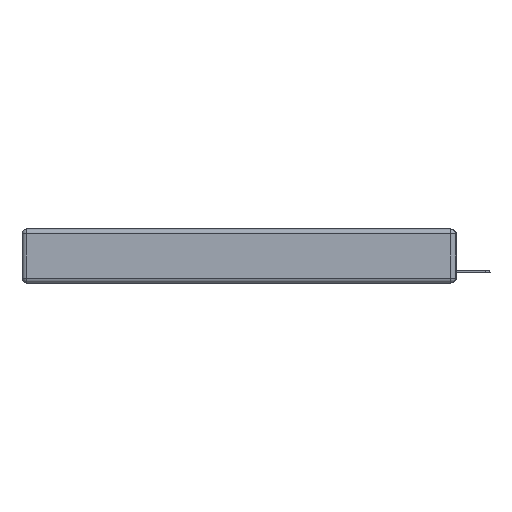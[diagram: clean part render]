
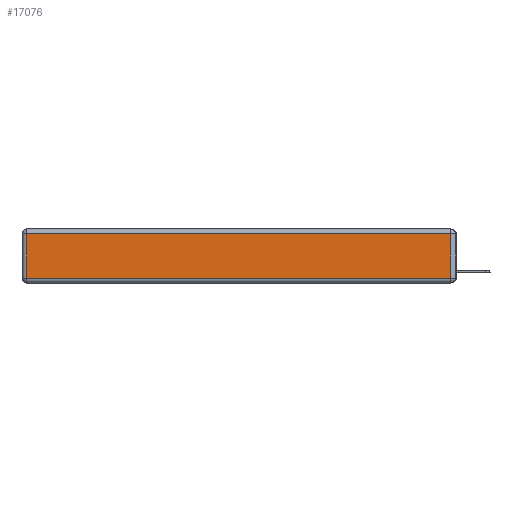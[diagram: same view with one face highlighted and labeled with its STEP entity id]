
A CAD part, left-side view. The second image highlights one B-rep face of the part: STEP entity #17076.
In plain terms, the highlighted planar face has unit normal (-1, 0, 0).
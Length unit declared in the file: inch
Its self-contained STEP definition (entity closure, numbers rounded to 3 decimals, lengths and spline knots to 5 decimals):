
#605 = CARTESIAN_POINT ( 'NONE',  ( 0., 2.72, -0.03 ) ) ;
#669 = EDGE_CURVE ( 'NONE', #10921, #11636, #18666, .T. ) ;
#800 = LINE ( 'NONE', #21331, #5895 ) ;
#1928 = LINE ( 'NONE', #9284, #22316 ) ;
#3323 = VECTOR ( 'NONE', #9651, 39.37008 ) ;
#4001 = DIRECTION ( 'NONE',  ( -1., 0., 0. ) ) ;
#5895 = VECTOR ( 'NONE', #8503, 39.37008 ) ;
#6489 = CARTESIAN_POINT ( 'NONE',  ( 0., 0.03, -0.313 ) ) ;
#7535 = EDGE_CURVE ( 'NONE', #11636, #9770, #1928, .T. ) ;
#7806 = LINE ( 'NONE', #19292, #3323 ) ;
#8338 = ORIENTED_EDGE ( 'NONE', *, *, #669, .T. ) ;
#8503 = DIRECTION ( 'NONE',  ( 0., 1., 0. ) ) ;
#9272 = CARTESIAN_POINT ( 'NONE',  ( 0., 0., -0.343 ) ) ;
#9284 = CARTESIAN_POINT ( 'NONE',  ( 0., 0.03, -0.343 ) ) ;
#9405 = DIRECTION ( 'NONE',  ( 0., 0., 1. ) ) ;
#9651 = DIRECTION ( 'NONE',  ( 0., 0., -1. ) ) ;
#9770 = VERTEX_POINT ( 'NONE', #18878 ) ;
#10065 = ORIENTED_EDGE ( 'NONE', *, *, #11985, .T. ) ;
#10921 = VERTEX_POINT ( 'NONE', #13803 ) ;
#11482 = DIRECTION ( 'NONE',  ( 0., 0., 1. ) ) ;
#11636 = VERTEX_POINT ( 'NONE', #6489 ) ;
#11985 = EDGE_CURVE ( 'NONE', #18352, #10921, #7806, .T. ) ;
#13312 = PLANE ( 'NONE',  #23325 ) ;
#13803 = CARTESIAN_POINT ( 'NONE',  ( 0., 2.72, -0.313 ) ) ;
#13859 = EDGE_CURVE ( 'NONE', #9770, #18352, #800, .T. ) ;
#15028 = FACE_OUTER_BOUND ( 'NONE', #21104, .T. ) ;
#17076 = ADVANCED_FACE ( 'NONE', ( #15028 ), #13312, .T. ) ;
#18352 = VERTEX_POINT ( 'NONE', #605 ) ;
#18666 = LINE ( 'NONE', #24018, #22579 ) ;
#18878 = CARTESIAN_POINT ( 'NONE',  ( 0., 0.03, -0.03 ) ) ;
#19292 = CARTESIAN_POINT ( 'NONE',  ( 0., 2.72, -0.343 ) ) ;
#20372 = DIRECTION ( 'NONE',  ( 0., -1., 0. ) ) ;
#21104 = EDGE_LOOP ( 'NONE', ( #8338, #22758, #22228, #10065 ) ) ;
#21331 = CARTESIAN_POINT ( 'NONE',  ( 0., 2.75, -0.03 ) ) ;
#22228 = ORIENTED_EDGE ( 'NONE', *, *, #13859, .T. ) ;
#22316 = VECTOR ( 'NONE', #9405, 39.37008 ) ;
#22579 = VECTOR ( 'NONE', #20372, 39.37008 ) ;
#22758 = ORIENTED_EDGE ( 'NONE', *, *, #7535, .T. ) ;
#23325 = AXIS2_PLACEMENT_3D ( 'NONE', #9272, #4001, #11482 ) ;
#24018 = CARTESIAN_POINT ( 'NONE',  ( 0., 0., -0.313 ) ) ;
